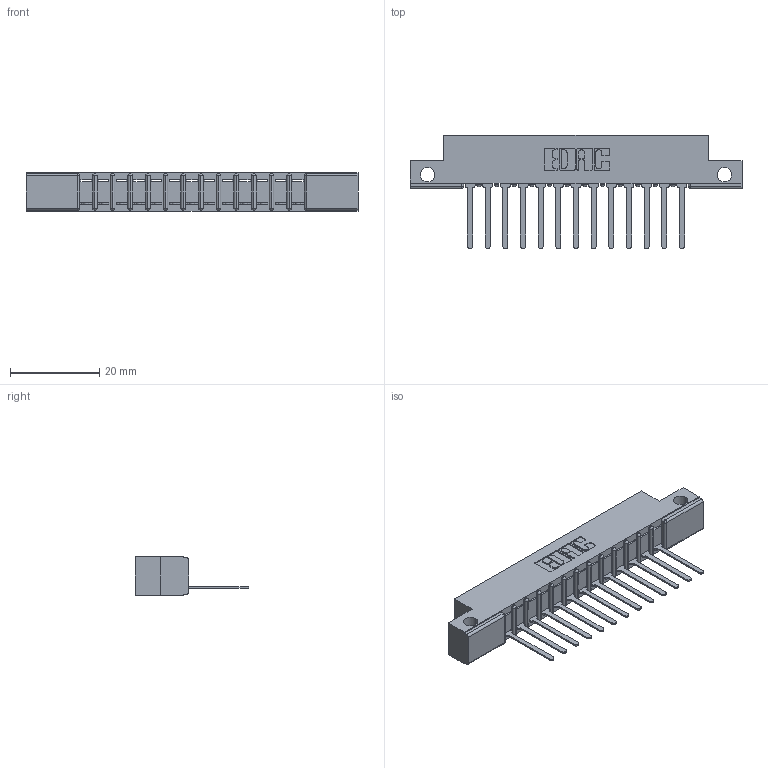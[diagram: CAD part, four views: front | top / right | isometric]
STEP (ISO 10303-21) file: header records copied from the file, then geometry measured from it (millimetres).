
FILE_DESCRIPTION (( 'STEP AP203' ), '1' );
FILE_NAME ('307-013-447-112.STEP', '2020-09-25T13:20:10', ( '' ), ( '' ), 'SwSTEP 2.0', 'SolidWorks 2020', '' );
FILE_SCHEMA (( 'CONFIG_CONTROL_DESIGN' ));
Length unit declared in the file: inch
Products named in the file (4): 307-290-001_547; 307-013-447-112; 307 Part_.128 Dia Side Mounting Holes; #16580
Assembly tree (14 placements, depth 2):
  307-013-447-112
    307 Part_.128 Dia Side Mounting Holes
    307-290-001_547  x13
  #16580
Bounding box: 74.52 x 25.43 x 8.71 mm (x, y, z)
Volume: 4681.7 mm3; surface area: 6947.8 mm2
Topology: 14 solids, 14 shells, 860 faces, 2429 edges, 1562 vertices
Faces by surface type: plane 551, cylinder 281, sphere 28
Entity records: 19509 total; most frequent: CARTESIAN_POINT 3245, ORIENTED_EDGE 3225, DIRECTION 3199, EDGE_CURVE 1604, LINE 1229, VECTOR 1220, VERTEX_POINT 1049, AXIS2_PLACEMENT_3D 988
